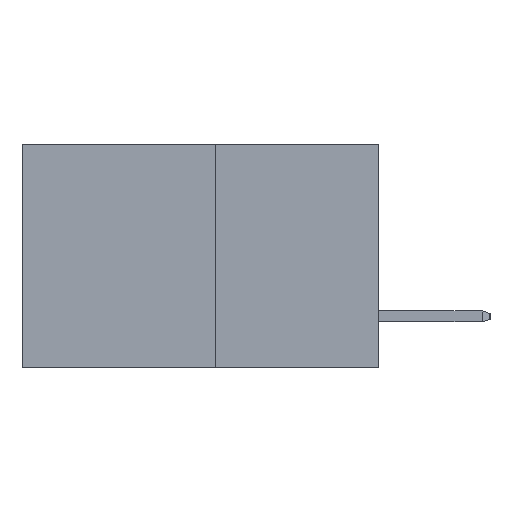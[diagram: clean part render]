
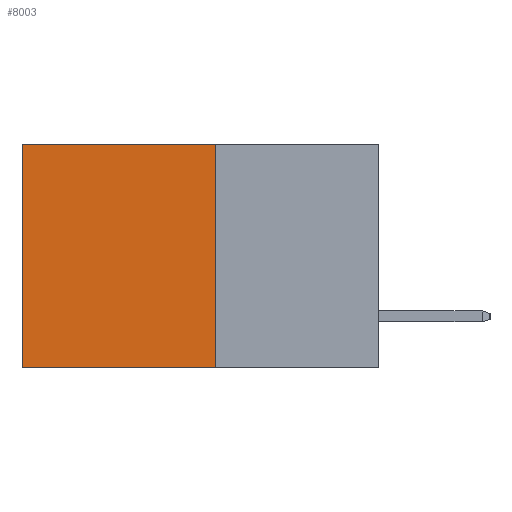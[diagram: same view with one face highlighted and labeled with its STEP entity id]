
A CAD part, left-side view. The second image highlights one B-rep face of the part: STEP entity #8003.
In plain terms, the highlighted planar face has unit normal (-1, 0, 0).
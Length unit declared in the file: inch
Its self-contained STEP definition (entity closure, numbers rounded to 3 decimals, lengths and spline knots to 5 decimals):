
#530 = CARTESIAN_POINT ( 'NONE',  ( 0.277, 0.27, 0. ) ) ;
#1346 = CARTESIAN_POINT ( 'NONE',  ( 0.277, 0.27, -0.37 ) ) ;
#3774 = CARTESIAN_POINT ( 'NONE',  ( 0.277, 0.27, -0.37 ) ) ;
#3907 = VERTEX_POINT ( 'NONE', #17726 ) ;
#4537 = DIRECTION ( 'NONE',  ( 0., 0., -1. ) ) ;
#4939 = LINE ( 'NONE', #5884, #17024 ) ;
#5768 = ORIENTED_EDGE ( 'NONE', *, *, #12055, .F. ) ;
#5884 = CARTESIAN_POINT ( 'NONE',  ( 0.277, 0.59, -0.37 ) ) ;
#7369 = CARTESIAN_POINT ( 'NONE',  ( 0.277, 0.27, -0.37 ) ) ;
#7487 = DIRECTION ( 'NONE',  ( 0., 0., -1. ) ) ;
#7750 = AXIS2_PLACEMENT_3D ( 'NONE', #1346, #14010, #4537 ) ;
#8003 = ADVANCED_FACE ( 'NONE', ( #16304 ), #12461, .F. ) ;
#8494 = LINE ( 'NONE', #3774, #12649 ) ;
#8682 = VECTOR ( 'NONE', #9033, 39.37008 ) ;
#9033 = DIRECTION ( 'NONE',  ( 0., 1., 0. ) ) ;
#9196 = VERTEX_POINT ( 'NONE', #12073 ) ;
#9568 = VERTEX_POINT ( 'NONE', #530 ) ;
#10526 = ORIENTED_EDGE ( 'NONE', *, *, #13481, .F. ) ;
#11708 = DIRECTION ( 'NONE',  ( 0., 0., -1. ) ) ;
#12055 = EDGE_CURVE ( 'NONE', #9568, #20045, #8494, .T. ) ;
#12073 = CARTESIAN_POINT ( 'NONE',  ( 0.277, 0.59, -0.37 ) ) ;
#12103 = DIRECTION ( 'NONE',  ( 0., 1., 0. ) ) ;
#12244 = EDGE_CURVE ( 'NONE', #3907, #9196, #4939, .T. ) ;
#12461 = PLANE ( 'NONE',  #7750 ) ;
#12649 = VECTOR ( 'NONE', #11708, 39.37008 ) ;
#12915 = CARTESIAN_POINT ( 'NONE',  ( 0.277, 0.27, -0.37 ) ) ;
#13481 = EDGE_CURVE ( 'NONE', #20045, #9196, #16970, .T. ) ;
#14010 = DIRECTION ( 'NONE',  ( 1., 0., 0. ) ) ;
#16029 = EDGE_CURVE ( 'NONE', #9568, #3907, #20318, .T. ) ;
#16270 = VECTOR ( 'NONE', #12103, 39.37008 ) ;
#16304 = FACE_OUTER_BOUND ( 'NONE', #17214, .T. ) ;
#16970 = LINE ( 'NONE', #7369, #8682 ) ;
#17024 = VECTOR ( 'NONE', #7487, 39.37008 ) ;
#17214 = EDGE_LOOP ( 'NONE', ( #20007, #10526, #5768, #18971 ) ) ;
#17726 = CARTESIAN_POINT ( 'NONE',  ( 0.277, 0.59, 0. ) ) ;
#18971 = ORIENTED_EDGE ( 'NONE', *, *, #16029, .T. ) ;
#19741 = CARTESIAN_POINT ( 'NONE',  ( 0.277, 0.27, 0. ) ) ;
#20007 = ORIENTED_EDGE ( 'NONE', *, *, #12244, .T. ) ;
#20045 = VERTEX_POINT ( 'NONE', #12915 ) ;
#20318 = LINE ( 'NONE', #19741, #16270 ) ;
